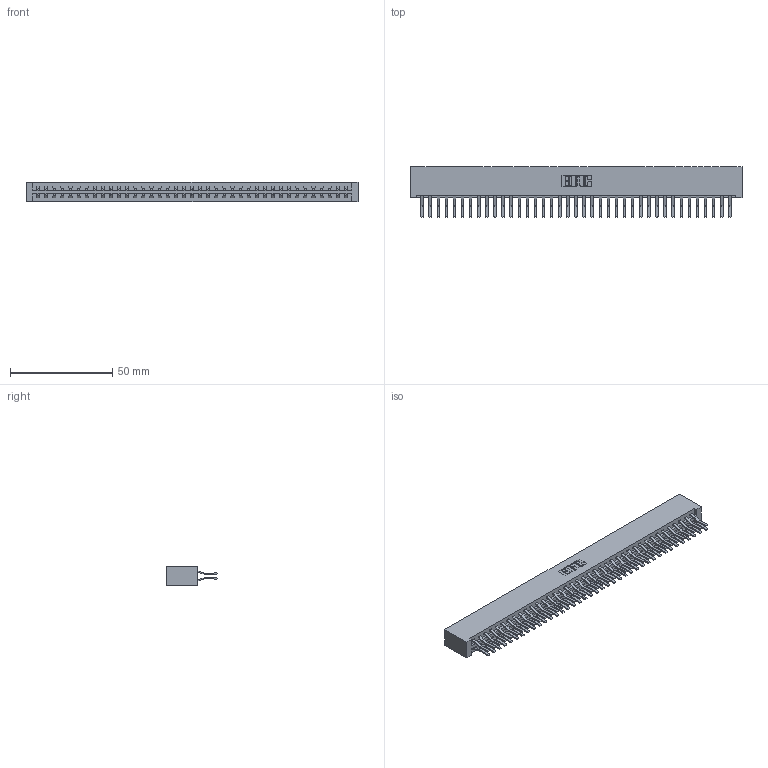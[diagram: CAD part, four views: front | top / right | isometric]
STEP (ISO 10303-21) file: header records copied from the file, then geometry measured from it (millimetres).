
FILE_DESCRIPTION (( 'STEP AP203' ), '1' );
FILE_NAME ('337-078-560-201.STEP', '2019-10-10T11:47:58', ( '' ), ( '' ), 'SwSTEP 2.0', 'SolidWorks 2016', '' );
FILE_SCHEMA (( 'CONFIG_CONTROL_DESIGN' ));
Length unit declared in the file: inch
Products named in the file (3): 337-078-560-201; 337 Part_No Mounting Lugs; 345-292-001_560 Tail
Assembly tree (79 placements, depth 2):
  337-078-560-201
    337 Part_No Mounting Lugs
    345-292-001_560 Tail  x78
Bounding box: 162.41 x 24.78 x 9.4 mm (x, y, z)
Volume: 18347.9 mm3; surface area: 22249 mm2
Topology: 79 solids, 79 shells, 4474 faces, 13313 edges, 8770 vertices
Faces by surface type: plane 3030, cylinder 1444
Entity records: 30437 total; most frequent: CARTESIAN_POINT 5130, ORIENTED_EDGE 5066, DIRECTION 4365, EDGE_CURVE 2533, LINE 2409, VECTOR 2409, VERTEX_POINT 1686, AXIS2_PLACEMENT_3D 978
